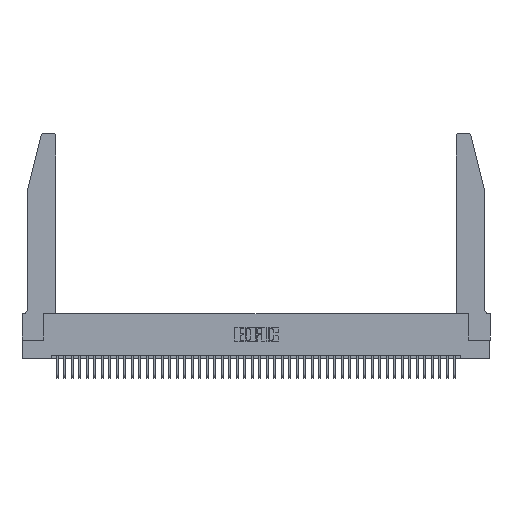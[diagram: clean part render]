
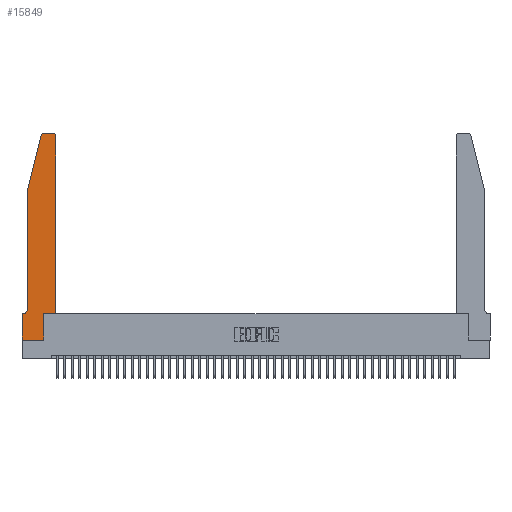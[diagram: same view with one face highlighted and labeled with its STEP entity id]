
A CAD part, top view. The second image highlights one B-rep face of the part: STEP entity #15849.
In plain terms, the highlighted planar face has unit normal (0, 0, 1).
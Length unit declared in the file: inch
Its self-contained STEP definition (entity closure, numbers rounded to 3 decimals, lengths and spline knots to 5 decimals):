
#533 = ORIENTED_EDGE ( 'NONE', *, *, #13136, .T. ) ;
#1835 = DIRECTION ( 'NONE',  ( 1., 0., 0. ) ) ;
#2804 = CARTESIAN_POINT ( 'NONE',  ( 0.2865, 0., 0.37 ) ) ;
#3187 = CARTESIAN_POINT ( 'NONE',  ( 0.4505, 0.35, 0.37 ) ) ;
#3971 = CARTESIAN_POINT ( 'NONE',  ( 0., 0.35, 0.37 ) ) ;
#4954 = VERTEX_POINT ( 'NONE', #14043 ) ;
#5199 = CARTESIAN_POINT ( 'NONE',  ( 0.0055, 0.35, 0.37 ) ) ;
#5480 = EDGE_CURVE ( 'NONE', #39366, #24763, #36826, .T. ) ;
#6068 = VECTOR ( 'NONE', #35309, 39.37008 ) ;
#6938 = AXIS2_PLACEMENT_3D ( 'NONE', #8519, #37383, #37531 ) ;
#7169 = DIRECTION ( 'NONE',  ( 0., 1., 0. ) ) ;
#7509 = EDGE_CURVE ( 'NONE', #23267, #28718, #18321, .T. ) ;
#8036 = DIRECTION ( 'NONE',  ( 0., -1., 0. ) ) ;
#8519 = CARTESIAN_POINT ( 'NONE',  ( 0., 0.35, 0.37 ) ) ;
#9235 = CARTESIAN_POINT ( 'NONE',  ( 0.4505, 2.72, 0.37 ) ) ;
#9340 = EDGE_CURVE ( 'NONE', #42375, #24917, #15842, .T. ) ;
#9853 = VECTOR ( 'NONE', #7169, 39.37008 ) ;
#10496 = ORIENTED_EDGE ( 'NONE', *, *, #44639, .T. ) ;
#12209 = PLANE ( 'NONE',  #6938 ) ;
#12385 = VERTEX_POINT ( 'NONE', #37467 ) ;
#12488 = CARTESIAN_POINT ( 'NONE',  ( 0.0055, 0.42, 0.37 ) ) ;
#12711 = CARTESIAN_POINT ( 'NONE',  ( 0.4505, 0.35, 0.37 ) ) ;
#13136 = EDGE_CURVE ( 'NONE', #4954, #15984, #41753, .T. ) ;
#13609 = CARTESIAN_POINT ( 'NONE',  ( 0., 0., 0.37 ) ) ;
#13660 = ORIENTED_EDGE ( 'NONE', *, *, #7509, .T. ) ;
#13936 = ORIENTED_EDGE ( 'NONE', *, *, #5480, .T. ) ;
#14012 = CARTESIAN_POINT ( 'NONE',  ( 0.25487, 2.72718, 0.37 ) ) ;
#14043 = CARTESIAN_POINT ( 'NONE',  ( 0.2865, 0.35, 0.37 ) ) ;
#14870 = DIRECTION ( 'NONE',  ( -1., 0., 0. ) ) ;
#15229 = CARTESIAN_POINT ( 'NONE',  ( 0.0755, 2., 0.37 ) ) ;
#15842 = LINE ( 'NONE', #13609, #6068 ) ;
#15849 = ADVANCED_FACE ( 'NONE', ( #44388 ), #12209, .T. ) ;
#15984 = VERTEX_POINT ( 'NONE', #20879 ) ;
#16171 = CARTESIAN_POINT ( 'NONE',  ( 0.0755, 0.35, 0.37 ) ) ;
#16198 = DIRECTION ( 'NONE',  ( -1., 0., 0. ) ) ;
#16305 = ORIENTED_EDGE ( 'NONE', *, *, #37667, .T. ) ;
#16418 = DIRECTION ( 'NONE',  ( 1., 0., 0. ) ) ;
#16830 = CARTESIAN_POINT ( 'NONE',  ( 0.0755, 2., 0.37 ) ) ;
#16952 = ORIENTED_EDGE ( 'NONE', *, *, #23517, .T. ) ;
#17087 = VECTOR ( 'NONE', #42051, 39.37008 ) ;
#17223 = DIRECTION ( 'NONE',  ( 0., 0., 1. ) ) ;
#17731 = DIRECTION ( 'NONE',  ( 0., -1., 0. ) ) ;
#18033 = DIRECTION ( 'NONE',  ( 0., 1., 0. ) ) ;
#18321 = LINE ( 'NONE', #18956, #45934 ) ;
#18956 = CARTESIAN_POINT ( 'NONE',  ( 0.0755, 2., 0.37 ) ) ;
#19605 = EDGE_CURVE ( 'NONE', #21397, #34225, #23391, .T. ) ;
#20115 = VECTOR ( 'NONE', #18033, 39.37008 ) ;
#20554 = ORIENTED_EDGE ( 'NONE', *, *, #19605, .T. ) ;
#20762 = LINE ( 'NONE', #29039, #9853 ) ;
#20879 = CARTESIAN_POINT ( 'NONE',  ( 0.4505, 0.35, 0.37 ) ) ;
#21397 = VERTEX_POINT ( 'NONE', #5199 ) ;
#23267 = VERTEX_POINT ( 'NONE', #15229 ) ;
#23391 = LINE ( 'NONE', #16171, #25928 ) ;
#23517 = EDGE_CURVE ( 'NONE', #46791, #23267, #32920, .T. ) ;
#23680 = CIRCLE ( 'NONE', #34051, 0.03 ) ;
#23950 = DIRECTION ( 'NONE',  ( 0., 0., 1. ) ) ;
#24763 = VERTEX_POINT ( 'NONE', #31150 ) ;
#24917 = VERTEX_POINT ( 'NONE', #2804 ) ;
#25928 = VECTOR ( 'NONE', #27149, 39.37008 ) ;
#27149 = DIRECTION ( 'NONE',  ( -1., 0., 0. ) ) ;
#28418 = EDGE_CURVE ( 'NONE', #28718, #21397, #34882, .T. ) ;
#28580 = CARTESIAN_POINT ( 'NONE',  ( 0.0755, 0.42, 0.37 ) ) ;
#28718 = VERTEX_POINT ( 'NONE', #28580 ) ;
#28798 = LINE ( 'NONE', #35724, #37175 ) ;
#29039 = CARTESIAN_POINT ( 'NONE',  ( 0.2865, 0.35, 0.37 ) ) ;
#30161 = EDGE_CURVE ( 'NONE', #24763, #12385, #31926, .T. ) ;
#31150 = CARTESIAN_POINT ( 'NONE',  ( 0.4205, 2.75, 0.37 ) ) ;
#31926 = LINE ( 'NONE', #43757, #40323 ) ;
#32920 = LINE ( 'NONE', #16830, #17087 ) ;
#34051 = AXIS2_PLACEMENT_3D ( 'NONE', #45438, #23950, #1835 ) ;
#34225 = VERTEX_POINT ( 'NONE', #3971 ) ;
#34487 = ORIENTED_EDGE ( 'NONE', *, *, #30161, .T. ) ;
#34882 = CIRCLE ( 'NONE', #46402, 0.07 ) ;
#35204 = CARTESIAN_POINT ( 'NONE',  ( 0., 0., 0.37 ) ) ;
#35309 = DIRECTION ( 'NONE',  ( 1., 0., 0. ) ) ;
#35724 = CARTESIAN_POINT ( 'NONE',  ( 0., 0., 0.37 ) ) ;
#36826 = CIRCLE ( 'NONE', #46335, 0.03 ) ;
#37175 = VECTOR ( 'NONE', #17731, 39.37008 ) ;
#37383 = DIRECTION ( 'NONE',  ( 0., 0., 1. ) ) ;
#37467 = CARTESIAN_POINT ( 'NONE',  ( 0.284, 2.75, 0.37 ) ) ;
#37531 = DIRECTION ( 'NONE',  ( 1., 0., 0. ) ) ;
#37667 = EDGE_CURVE ( 'NONE', #34225, #42375, #28798, .T. ) ;
#37809 = DIRECTION ( 'NONE',  ( 0., 0., -1. ) ) ;
#38008 = EDGE_CURVE ( 'NONE', #12385, #46791, #23680, .T. ) ;
#38836 = CARTESIAN_POINT ( 'NONE',  ( 0.4205, 2.72, 0.37 ) ) ;
#39366 = VERTEX_POINT ( 'NONE', #9235 ) ;
#40323 = VECTOR ( 'NONE', #14870, 39.37008 ) ;
#40395 = LINE ( 'NONE', #3187, #20115 ) ;
#40614 = VECTOR ( 'NONE', #16418, 39.37008 ) ;
#41614 = ORIENTED_EDGE ( 'NONE', *, *, #44014, .T. ) ;
#41753 = LINE ( 'NONE', #12711, #40614 ) ;
#42051 = DIRECTION ( 'NONE',  ( -0.239, -0.971, 0. ) ) ;
#42340 = ORIENTED_EDGE ( 'NONE', *, *, #9340, .T. ) ;
#42375 = VERTEX_POINT ( 'NONE', #35204 ) ;
#42466 = DIRECTION ( 'NONE',  ( 1., 0., 0. ) ) ;
#43757 = CARTESIAN_POINT ( 'NONE',  ( 0.2605, 2.75, 0.37 ) ) ;
#44014 = EDGE_CURVE ( 'NONE', #24917, #4954, #20762, .T. ) ;
#44388 = FACE_OUTER_BOUND ( 'NONE', #45403, .T. ) ;
#44639 = EDGE_CURVE ( 'NONE', #15984, #39366, #40395, .T. ) ;
#45403 = EDGE_LOOP ( 'NONE', ( #34487, #45705, #16952, #13660, #46993, #20554, #16305, #42340, #41614, #533, #10496, #13936 ) ) ;
#45438 = CARTESIAN_POINT ( 'NONE',  ( 0.284, 2.72, 0.37 ) ) ;
#45705 = ORIENTED_EDGE ( 'NONE', *, *, #38008, .T. ) ;
#45934 = VECTOR ( 'NONE', #8036, 39.37008 ) ;
#46335 = AXIS2_PLACEMENT_3D ( 'NONE', #38836, #17223, #42466 ) ;
#46402 = AXIS2_PLACEMENT_3D ( 'NONE', #12488, #37809, #16198 ) ;
#46791 = VERTEX_POINT ( 'NONE', #14012 ) ;
#46993 = ORIENTED_EDGE ( 'NONE', *, *, #28418, .T. ) ;
